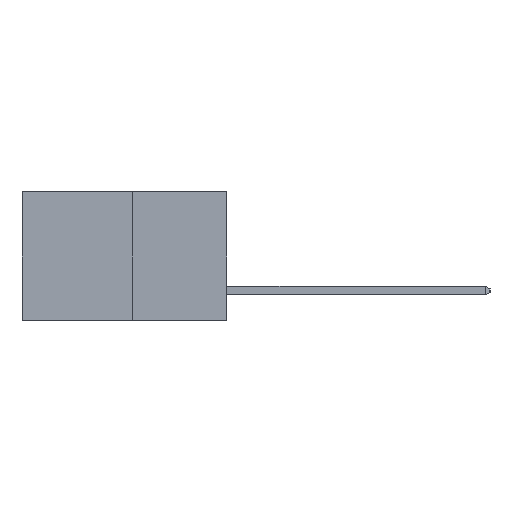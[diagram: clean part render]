
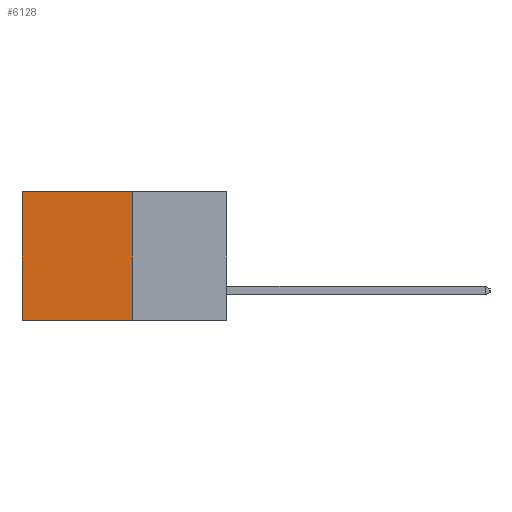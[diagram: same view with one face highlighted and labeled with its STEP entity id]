
A CAD part, left-side view. The second image highlights one B-rep face of the part: STEP entity #6128.
In plain terms, the highlighted planar face has unit normal (-1, 0, 0).
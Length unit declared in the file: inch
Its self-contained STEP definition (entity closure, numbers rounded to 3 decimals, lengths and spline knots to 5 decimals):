
#50 = VERTEX_POINT ( 'NONE', #7733 ) ;
#286 = VERTEX_POINT ( 'NONE', #2396 ) ;
#418 = CARTESIAN_POINT ( 'NONE',  ( 0.277, 0.59, 0. ) ) ;
#561 = EDGE_CURVE ( 'NONE', #1431, #50, #8284, .T. ) ;
#690 = LINE ( 'NONE', #6030, #8728 ) ;
#762 = ORIENTED_EDGE ( 'NONE', *, *, #3472, .F. ) ;
#1431 = VERTEX_POINT ( 'NONE', #10250 ) ;
#2396 = CARTESIAN_POINT ( 'NONE',  ( 0.277, 0.59, -0.37 ) ) ;
#2700 = LINE ( 'NONE', #10318, #4840 ) ;
#3301 = CARTESIAN_POINT ( 'NONE',  ( 0.277, 0.27, -0.37 ) ) ;
#3472 = EDGE_CURVE ( 'NONE', #50, #286, #2700, .T. ) ;
#3627 = DIRECTION ( 'NONE',  ( 0., 0., -1. ) ) ;
#3828 = VECTOR ( 'NONE', #6543, 39.37008 ) ;
#3858 = EDGE_CURVE ( 'NONE', #1431, #4791, #690, .T. ) ;
#4146 = ORIENTED_EDGE ( 'NONE', *, *, #3858, .T. ) ;
#4702 = LINE ( 'NONE', #9110, #6752 ) ;
#4791 = VERTEX_POINT ( 'NONE', #418 ) ;
#4840 = VECTOR ( 'NONE', #7804, 39.37008 ) ;
#5960 = ORIENTED_EDGE ( 'NONE', *, *, #9582, .T. ) ;
#6030 = CARTESIAN_POINT ( 'NONE',  ( 0.277, 0.27, 0. ) ) ;
#6128 = ADVANCED_FACE ( 'NONE', ( #9729 ), #7090, .F. ) ;
#6543 = DIRECTION ( 'NONE',  ( 0., 0., -1. ) ) ;
#6604 = DIRECTION ( 'NONE',  ( 0., 1., 0. ) ) ;
#6752 = VECTOR ( 'NONE', #3627, 39.37008 ) ;
#6825 = DIRECTION ( 'NONE',  ( 0., 0., -1. ) ) ;
#6882 = DIRECTION ( 'NONE',  ( 1., 0., 0. ) ) ;
#6928 = EDGE_LOOP ( 'NONE', ( #5960, #762, #10063, #4146 ) ) ;
#7090 = PLANE ( 'NONE',  #8631 ) ;
#7733 = CARTESIAN_POINT ( 'NONE',  ( 0.277, 0.27, -0.37 ) ) ;
#7804 = DIRECTION ( 'NONE',  ( 0., 1., 0. ) ) ;
#8284 = LINE ( 'NONE', #3301, #3828 ) ;
#8631 = AXIS2_PLACEMENT_3D ( 'NONE', #8988, #6882, #6825 ) ;
#8728 = VECTOR ( 'NONE', #6604, 39.37008 ) ;
#8988 = CARTESIAN_POINT ( 'NONE',  ( 0.277, 0.27, -0.37 ) ) ;
#9110 = CARTESIAN_POINT ( 'NONE',  ( 0.277, 0.59, -0.37 ) ) ;
#9582 = EDGE_CURVE ( 'NONE', #4791, #286, #4702, .T. ) ;
#9729 = FACE_OUTER_BOUND ( 'NONE', #6928, .T. ) ;
#10063 = ORIENTED_EDGE ( 'NONE', *, *, #561, .F. ) ;
#10250 = CARTESIAN_POINT ( 'NONE',  ( 0.277, 0.27, 0. ) ) ;
#10318 = CARTESIAN_POINT ( 'NONE',  ( 0.277, 0.27, -0.37 ) ) ;
